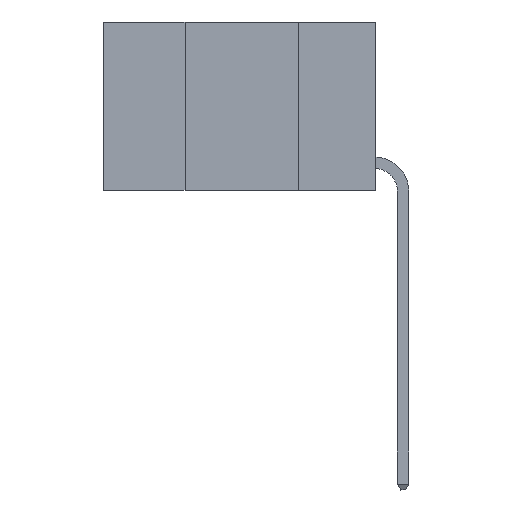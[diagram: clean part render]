
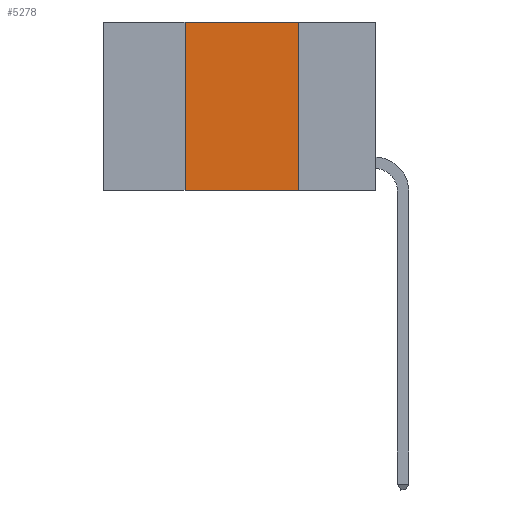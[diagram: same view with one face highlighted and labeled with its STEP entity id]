
A CAD part, left-side view. The second image highlights one B-rep face of the part: STEP entity #5278.
In plain terms, the highlighted planar face has unit normal (-1, 0, 0).
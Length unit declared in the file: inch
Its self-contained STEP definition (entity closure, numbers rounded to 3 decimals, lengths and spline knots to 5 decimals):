
#177 = LINE ( 'NONE', #9353, #28632 ) ;
#338 = VECTOR ( 'NONE', #11353, 39.37008 ) ;
#1025 = VERTEX_POINT ( 'NONE', #29226 ) ;
#4299 = CARTESIAN_POINT ( 'NONE',  ( 0., 0.6, -0.37 ) ) ;
#4535 = DIRECTION ( 'NONE',  ( 0., 0., 1. ) ) ;
#4989 = DIRECTION ( 'NONE',  ( 0., -1., 0. ) ) ;
#5278 = ADVANCED_FACE ( 'NONE', ( #17346 ), #20033, .F. ) ;
#5425 = VERTEX_POINT ( 'NONE', #18392 ) ;
#6803 = CARTESIAN_POINT ( 'NONE',  ( 0., 0.42, 0. ) ) ;
#7024 = DIRECTION ( 'NONE',  ( 0., 0., -1. ) ) ;
#9221 = ORIENTED_EDGE ( 'NONE', *, *, #21134, .T. ) ;
#9353 = CARTESIAN_POINT ( 'NONE',  ( 0., 0.6, 0. ) ) ;
#10311 = CARTESIAN_POINT ( 'NONE',  ( 0., 0.6, 0. ) ) ;
#11209 = LINE ( 'NONE', #4299, #338 ) ;
#11353 = DIRECTION ( 'NONE',  ( 0., -1., 0. ) ) ;
#11515 = LINE ( 'NONE', #27539, #28196 ) ;
#12240 = VERTEX_POINT ( 'NONE', #23002 ) ;
#12553 = DIRECTION ( 'NONE',  ( 0., 0., -1. ) ) ;
#14108 = ORIENTED_EDGE ( 'NONE', *, *, #24250, .F. ) ;
#15101 = DIRECTION ( 'NONE',  ( 1., 0., 0. ) ) ;
#17346 = FACE_OUTER_BOUND ( 'NONE', #25211, .T. ) ;
#17943 = ORIENTED_EDGE ( 'NONE', *, *, #25279, .F. ) ;
#18392 = CARTESIAN_POINT ( 'NONE',  ( 0., 0.42, 0. ) ) ;
#20033 = PLANE ( 'NONE',  #27979 ) ;
#20102 = ORIENTED_EDGE ( 'NONE', *, *, #23376, .F. ) ;
#21134 = EDGE_CURVE ( 'NONE', #12240, #1025, #11209, .T. ) ;
#21931 = VECTOR ( 'NONE', #4535, 39.37008 ) ;
#22331 = VERTEX_POINT ( 'NONE', #24834 ) ;
#23002 = CARTESIAN_POINT ( 'NONE',  ( 0., 0.42, -0.37 ) ) ;
#23270 = LINE ( 'NONE', #6803, #21931 ) ;
#23376 = EDGE_CURVE ( 'NONE', #12240, #5425, #23270, .T. ) ;
#24250 = EDGE_CURVE ( 'NONE', #5425, #22331, #177, .T. ) ;
#24834 = CARTESIAN_POINT ( 'NONE',  ( 0., 0.17, 0. ) ) ;
#25211 = EDGE_LOOP ( 'NONE', ( #17943, #14108, #20102, #9221 ) ) ;
#25279 = EDGE_CURVE ( 'NONE', #22331, #1025, #11515, .T. ) ;
#27539 = CARTESIAN_POINT ( 'NONE',  ( 0., 0.17, 0. ) ) ;
#27979 = AXIS2_PLACEMENT_3D ( 'NONE', #10311, #15101, #12553 ) ;
#28196 = VECTOR ( 'NONE', #7024, 39.37008 ) ;
#28632 = VECTOR ( 'NONE', #4989, 39.37008 ) ;
#29226 = CARTESIAN_POINT ( 'NONE',  ( 0., 0.17, -0.37 ) ) ;
